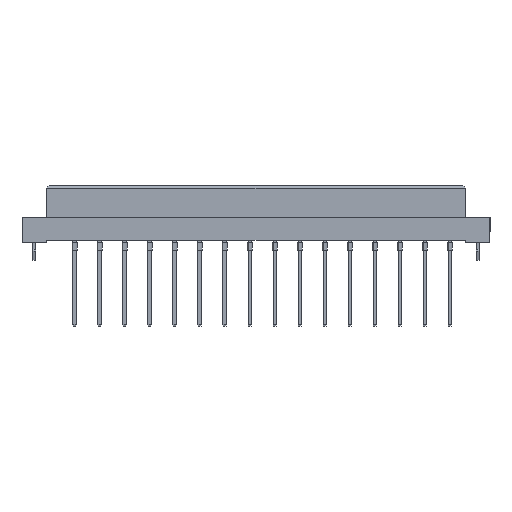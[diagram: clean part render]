
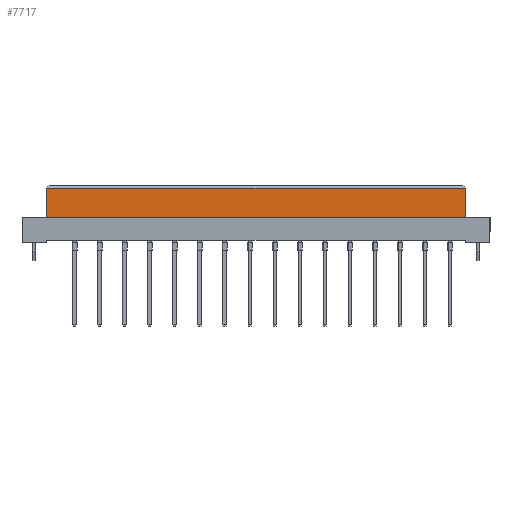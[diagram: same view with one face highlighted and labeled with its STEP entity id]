
A CAD part, top view. The second image highlights one B-rep face of the part: STEP entity #7717.
In plain terms, the highlighted planar face has unit normal (0, 0, 1).
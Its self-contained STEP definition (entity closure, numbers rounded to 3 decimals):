
#112 = EDGE_CURVE ( 'NONE', #27857, #15395, #24226, .T. ) ;
#864 = DIRECTION ( 'NONE',  ( 0., 1., 0. ) ) ;
#3467 = EDGE_CURVE ( 'NONE', #27857, #9935, #10703, .T. ) ;
#4799 = LINE ( 'NONE', #35654, #20088 ) ;
#5481 = DIRECTION ( 'NONE',  ( 0., 0., 1. ) ) ;
#6698 = AXIS2_PLACEMENT_3D ( 'NONE', #29234, #5481, #32001 ) ;
#7389 = CARTESIAN_POINT ( 'NONE',  ( 42.5, -6.4, 4.25 ) ) ;
#7717 = ADVANCED_FACE ( 'NONE', ( #26279 ), #17177, .T. ) ;
#9935 = VERTEX_POINT ( 'NONE', #37352 ) ;
#10703 = LINE ( 'NONE', #37035, #23417 ) ;
#10839 = EDGE_CURVE ( 'NONE', #15395, #16821, #25207, .T. ) ;
#14850 = EDGE_CURVE ( 'NONE', #16821, #9935, #4799, .T. ) ;
#15248 = VECTOR ( 'NONE', #864, 1000. ) ;
#15395 = VERTEX_POINT ( 'NONE', #34427 ) ;
#15416 = ORIENTED_EDGE ( 'NONE', *, *, #14850, .T. ) ;
#16821 = VERTEX_POINT ( 'NONE', #27296 ) ;
#17177 = PLANE ( 'NONE',  #6698 ) ;
#19040 = DIRECTION ( 'NONE',  ( 0., 1., 0. ) ) ;
#20088 = VECTOR ( 'NONE', #20243, 1000. ) ;
#20138 = EDGE_LOOP ( 'NONE', ( #31156, #15416, #22251, #22603 ) ) ;
#20243 = DIRECTION ( 'NONE',  ( -1., 0., 0. ) ) ;
#22251 = ORIENTED_EDGE ( 'NONE', *, *, #3467, .F. ) ;
#22603 = ORIENTED_EDGE ( 'NONE', *, *, #112, .T. ) ;
#23417 = VECTOR ( 'NONE', #19040, 1000. ) ;
#24226 = LINE ( 'NONE', #32003, #25285 ) ;
#25207 = LINE ( 'NONE', #7389, #15248 ) ;
#25285 = VECTOR ( 'NONE', #26990, 1000. ) ;
#26279 = FACE_OUTER_BOUND ( 'NONE', #20138, .T. ) ;
#26990 = DIRECTION ( 'NONE',  ( 1., 0., 0. ) ) ;
#27296 = CARTESIAN_POINT ( 'NONE',  ( 42.5, -0.5, 4.25 ) ) ;
#27857 = VERTEX_POINT ( 'NONE', #32934 ) ;
#29234 = CARTESIAN_POINT ( 'NONE',  ( 42.5, -6.4, 4.25 ) ) ;
#31156 = ORIENTED_EDGE ( 'NONE', *, *, #10839, .T. ) ;
#32001 = DIRECTION ( 'NONE',  ( 1., 0., 0. ) ) ;
#32003 = CARTESIAN_POINT ( 'NONE',  ( 42.5, -6.4, 4.25 ) ) ;
#32934 = CARTESIAN_POINT ( 'NONE',  ( -42.5, -6.4, 4.25 ) ) ;
#34427 = CARTESIAN_POINT ( 'NONE',  ( 42.5, -6.4, 4.25 ) ) ;
#35654 = CARTESIAN_POINT ( 'NONE',  ( -42.5, -0.5, 4.25 ) ) ;
#37035 = CARTESIAN_POINT ( 'NONE',  ( -42.5, -6.4, 4.25 ) ) ;
#37352 = CARTESIAN_POINT ( 'NONE',  ( -42.5, -0.5, 4.25 ) ) ;
